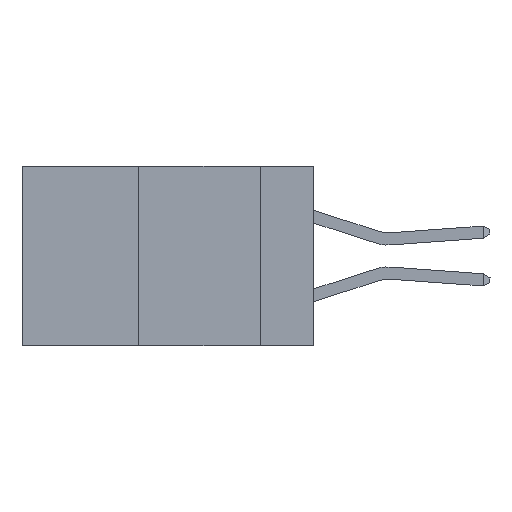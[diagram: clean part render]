
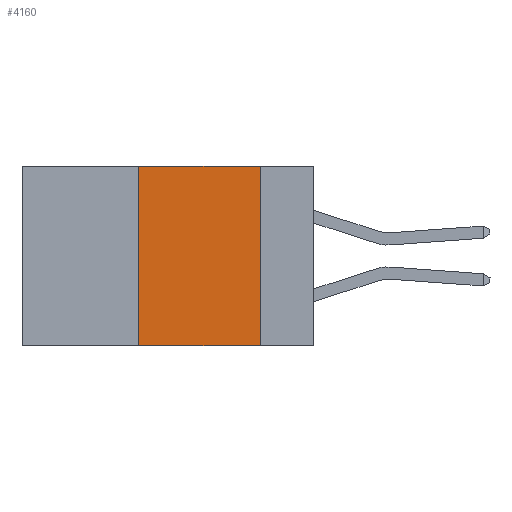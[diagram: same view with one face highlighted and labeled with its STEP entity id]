
A CAD part, left-side view. The second image highlights one B-rep face of the part: STEP entity #4160.
In plain terms, the highlighted planar face has unit normal (-1, 0, 0).
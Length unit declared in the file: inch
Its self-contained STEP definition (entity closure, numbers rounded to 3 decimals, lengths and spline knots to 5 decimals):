
#566 = ORIENTED_EDGE ( 'NONE', *, *, #5879, .F. ) ;
#903 = DIRECTION ( 'NONE',  ( 0., 0., -1. ) ) ;
#2146 = CARTESIAN_POINT ( 'NONE',  ( 0., 0.11, -0.37 ) ) ;
#2332 = LINE ( 'NONE', #9506, #9938 ) ;
#2595 = VECTOR ( 'NONE', #3303, 39.37008 ) ;
#2936 = ORIENTED_EDGE ( 'NONE', *, *, #6387, .F. ) ;
#2966 = VERTEX_POINT ( 'NONE', #9706 ) ;
#3303 = DIRECTION ( 'NONE',  ( 0., 0., 1. ) ) ;
#3777 = EDGE_CURVE ( 'NONE', #2966, #8235, #8848, .T. ) ;
#3946 = CARTESIAN_POINT ( 'NONE',  ( 0., 0.36, 0. ) ) ;
#4160 = ADVANCED_FACE ( 'NONE', ( #4294 ), #8514, .F. ) ;
#4294 = FACE_OUTER_BOUND ( 'NONE', #4948, .T. ) ;
#4310 = DIRECTION ( 'NONE',  ( 0., -1., 0. ) ) ;
#4948 = EDGE_LOOP ( 'NONE', ( #566, #5268, #2936, #5185 ) ) ;
#5183 = DIRECTION ( 'NONE',  ( 0., 0., -1. ) ) ;
#5185 = ORIENTED_EDGE ( 'NONE', *, *, #10967, .T. ) ;
#5268 = ORIENTED_EDGE ( 'NONE', *, *, #3777, .F. ) ;
#5634 = CARTESIAN_POINT ( 'NONE',  ( 0., 0.11, 0. ) ) ;
#5879 = EDGE_CURVE ( 'NONE', #8235, #9715, #12882, .T. ) ;
#5923 = VECTOR ( 'NONE', #4310, 39.37008 ) ;
#6387 = EDGE_CURVE ( 'NONE', #13871, #2966, #12141, .T. ) ;
#8126 = CARTESIAN_POINT ( 'NONE',  ( 0., 0.11, 0. ) ) ;
#8235 = VERTEX_POINT ( 'NONE', #8126 ) ;
#8514 = PLANE ( 'NONE',  #11972 ) ;
#8848 = LINE ( 'NONE', #13586, #5923 ) ;
#9051 = DIRECTION ( 'NONE',  ( 0., -1., 0. ) ) ;
#9506 = CARTESIAN_POINT ( 'NONE',  ( 0., 0.6, -0.37 ) ) ;
#9706 = CARTESIAN_POINT ( 'NONE',  ( 0., 0.36, 0. ) ) ;
#9715 = VERTEX_POINT ( 'NONE', #2146 ) ;
#9820 = CARTESIAN_POINT ( 'NONE',  ( 0., 0.6, 0. ) ) ;
#9938 = VECTOR ( 'NONE', #9051, 39.37008 ) ;
#10967 = EDGE_CURVE ( 'NONE', #13871, #9715, #2332, .T. ) ;
#11972 = AXIS2_PLACEMENT_3D ( 'NONE', #9820, #11996, #5183 ) ;
#11996 = DIRECTION ( 'NONE',  ( 1., 0., 0. ) ) ;
#12141 = LINE ( 'NONE', #3946, #2595 ) ;
#12882 = LINE ( 'NONE', #5634, #14576 ) ;
#13586 = CARTESIAN_POINT ( 'NONE',  ( 0., 0.6, 0. ) ) ;
#13871 = VERTEX_POINT ( 'NONE', #14643 ) ;
#14576 = VECTOR ( 'NONE', #903, 39.37008 ) ;
#14643 = CARTESIAN_POINT ( 'NONE',  ( 0., 0.36, -0.37 ) ) ;
